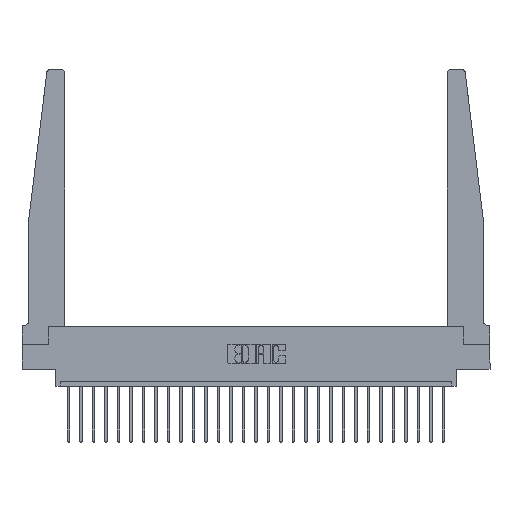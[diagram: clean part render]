
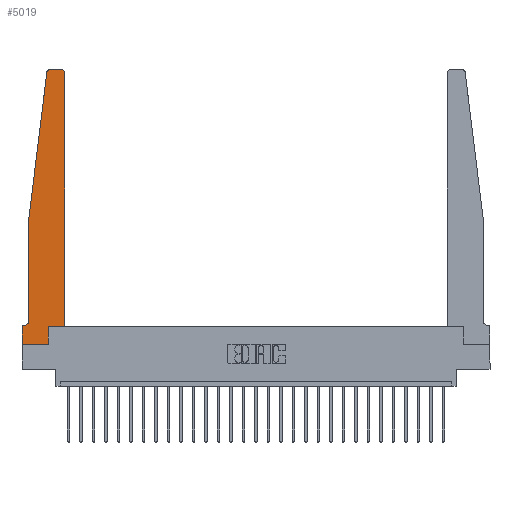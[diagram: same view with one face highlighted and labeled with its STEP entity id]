
A CAD part, top view. The second image highlights one B-rep face of the part: STEP entity #5019.
In plain terms, the highlighted planar face has unit normal (0, 0, 1).
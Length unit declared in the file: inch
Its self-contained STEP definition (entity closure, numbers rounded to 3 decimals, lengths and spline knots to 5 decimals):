
#34 = CARTESIAN_POINT ( 'NONE',  ( 0.065, 1.25, 0.37 ) ) ;
#147 = EDGE_CURVE ( 'NONE', #15718, #2009, #24864, .T. ) ;
#319 = DIRECTION ( 'NONE',  ( 1., 0., 0. ) ) ;
#338 = CARTESIAN_POINT ( 'NONE',  ( 0.425, 0.18, 0.37 ) ) ;
#921 = CARTESIAN_POINT ( 'NONE',  ( 0.2605, 0.18, 0.37 ) ) ;
#945 = EDGE_CURVE ( 'NONE', #9251, #15557, #10658, .T. ) ;
#1356 = VERTEX_POINT ( 'NONE', #6340 ) ;
#1783 = CARTESIAN_POINT ( 'NONE',  ( 0.395, 2.72, 0.37 ) ) ;
#2009 = VERTEX_POINT ( 'NONE', #18451 ) ;
#2066 = CARTESIAN_POINT ( 'NONE',  ( 0., 0., 0.37 ) ) ;
#2299 = DIRECTION ( 'NONE',  ( 0., 1., 0. ) ) ;
#2310 = AXIS2_PLACEMENT_3D ( 'NONE', #1783, #15769, #21494 ) ;
#2678 = EDGE_CURVE ( 'NONE', #15557, #17619, #13947, .T. ) ;
#3442 = EDGE_CURVE ( 'NONE', #2009, #15219, #23476, .T. ) ;
#3740 = LINE ( 'NONE', #34, #7830 ) ;
#4652 = VERTEX_POINT ( 'NONE', #17534 ) ;
#5019 = ADVANCED_FACE ( 'NONE', ( #23372 ), #10019, .T. ) ;
#5149 = VECTOR ( 'NONE', #2299, 39.37008 ) ;
#5150 = CARTESIAN_POINT ( 'NONE',  ( 0.2605, 0.18, 0.37 ) ) ;
#5311 = CARTESIAN_POINT ( 'NONE',  ( 0.015, 0.2375, 0.37 ) ) ;
#5562 = DIRECTION ( 'NONE',  ( 0., -1., 0. ) ) ;
#5778 = CARTESIAN_POINT ( 'NONE',  ( 0.2605, 0., 0.37 ) ) ;
#6340 = CARTESIAN_POINT ( 'NONE',  ( 0.015, 0.1875, 0.37 ) ) ;
#6623 = ORIENTED_EDGE ( 'NONE', *, *, #3442, .T. ) ;
#6877 = VECTOR ( 'NONE', #22052, 39.37008 ) ;
#6918 = CARTESIAN_POINT ( 'NONE',  ( 0.24675, 2.72367, 0.37 ) ) ;
#7830 = VECTOR ( 'NONE', #21625, 39.37008 ) ;
#8407 = ORIENTED_EDGE ( 'NONE', *, *, #9617, .T. ) ;
#8444 = ORIENTED_EDGE ( 'NONE', *, *, #14820, .T. ) ;
#8614 = VECTOR ( 'NONE', #23324, 39.37008 ) ;
#8961 = CIRCLE ( 'NONE', #15081, 0.03 ) ;
#9251 = VERTEX_POINT ( 'NONE', #17848 ) ;
#9331 = VERTEX_POINT ( 'NONE', #10132 ) ;
#9617 = EDGE_CURVE ( 'NONE', #18121, #9331, #22500, .T. ) ;
#9784 = CARTESIAN_POINT ( 'NONE',  ( 0., 0., 0.37 ) ) ;
#9858 = ORIENTED_EDGE ( 'NONE', *, *, #20325, .T. ) ;
#10019 = PLANE ( 'NONE',  #12121 ) ;
#10081 = DIRECTION ( 'NONE',  ( -1., 0., 0. ) ) ;
#10132 = CARTESIAN_POINT ( 'NONE',  ( 0.065, 0.2375, 0.37 ) ) ;
#10326 = CARTESIAN_POINT ( 'NONE',  ( 0.065, 0.1875, 0.37 ) ) ;
#10343 = LINE ( 'NONE', #24431, #23898 ) ;
#10490 = CIRCLE ( 'NONE', #2310, 0.03 ) ;
#10658 = LINE ( 'NONE', #2066, #15305 ) ;
#10981 = ORIENTED_EDGE ( 'NONE', *, *, #12804, .T. ) ;
#11091 = DIRECTION ( 'NONE',  ( 0., 1., 0. ) ) ;
#12029 = CARTESIAN_POINT ( 'NONE',  ( 0., 0.1875, 0.37 ) ) ;
#12121 = AXIS2_PLACEMENT_3D ( 'NONE', #12029, #14042, #319 ) ;
#12804 = EDGE_CURVE ( 'NONE', #15863, #4652, #10343, .T. ) ;
#12866 = EDGE_CURVE ( 'NONE', #18465, #18121, #3740, .T. ) ;
#13024 = EDGE_CURVE ( 'NONE', #1356, #9251, #24803, .T. ) ;
#13165 = CARTESIAN_POINT ( 'NONE',  ( 0.27653, 2.72, 0.37 ) ) ;
#13483 = DIRECTION ( 'NONE',  ( 0., 0., -1. ) ) ;
#13665 = CARTESIAN_POINT ( 'NONE',  ( 0.065, 1.25, 0.37 ) ) ;
#13947 = LINE ( 'NONE', #9784, #8614 ) ;
#14042 = DIRECTION ( 'NONE',  ( 0., 0., 1. ) ) ;
#14306 = ORIENTED_EDGE ( 'NONE', *, *, #24578, .T. ) ;
#14345 = CARTESIAN_POINT ( 'NONE',  ( 0.395, 2.75, 0.37 ) ) ;
#14661 = VECTOR ( 'NONE', #20088, 39.37008 ) ;
#14820 = EDGE_CURVE ( 'NONE', #9331, #1356, #14877, .T. ) ;
#14877 = CIRCLE ( 'NONE', #23794, 0.05 ) ;
#14976 = DIRECTION ( 'NONE',  ( 0., 0., 1. ) ) ;
#15081 = AXIS2_PLACEMENT_3D ( 'NONE', #13165, #14976, #24588 ) ;
#15219 = VERTEX_POINT ( 'NONE', #16617 ) ;
#15278 = EDGE_CURVE ( 'NONE', #4652, #18465, #8961, .T. ) ;
#15305 = VECTOR ( 'NONE', #16053, 39.37008 ) ;
#15557 = VERTEX_POINT ( 'NONE', #18737 ) ;
#15718 = VERTEX_POINT ( 'NONE', #5150 ) ;
#15769 = DIRECTION ( 'NONE',  ( 0., 0., 1. ) ) ;
#15863 = VERTEX_POINT ( 'NONE', #14345 ) ;
#16053 = DIRECTION ( 'NONE',  ( 0., -1., 0. ) ) ;
#16617 = CARTESIAN_POINT ( 'NONE',  ( 0.425, 2.72, 0.37 ) ) ;
#17170 = EDGE_LOOP ( 'NONE', ( #10981, #18918, #18441, #8407, #8444, #24070, #21725, #21412, #9858, #20724, #6623, #14306 ) ) ;
#17534 = CARTESIAN_POINT ( 'NONE',  ( 0.27653, 2.75, 0.37 ) ) ;
#17619 = VERTEX_POINT ( 'NONE', #5778 ) ;
#17848 = CARTESIAN_POINT ( 'NONE',  ( 0., 0.1875, 0.37 ) ) ;
#18121 = VERTEX_POINT ( 'NONE', #21440 ) ;
#18441 = ORIENTED_EDGE ( 'NONE', *, *, #12866, .T. ) ;
#18451 = CARTESIAN_POINT ( 'NONE',  ( 0.425, 0.18, 0.37 ) ) ;
#18465 = VERTEX_POINT ( 'NONE', #6918 ) ;
#18737 = CARTESIAN_POINT ( 'NONE',  ( 0., 0., 0.37 ) ) ;
#18918 = ORIENTED_EDGE ( 'NONE', *, *, #15278, .T. ) ;
#19005 = DIRECTION ( 'NONE',  ( -1., 0., 0. ) ) ;
#19996 = CARTESIAN_POINT ( 'NONE',  ( 0.425, 0.18, 0.37 ) ) ;
#20035 = VECTOR ( 'NONE', #5562, 39.37008 ) ;
#20088 = DIRECTION ( 'NONE',  ( -1., 0., 0. ) ) ;
#20325 = EDGE_CURVE ( 'NONE', #17619, #15718, #22089, .T. ) ;
#20724 = ORIENTED_EDGE ( 'NONE', *, *, #147, .T. ) ;
#21412 = ORIENTED_EDGE ( 'NONE', *, *, #2678, .T. ) ;
#21440 = CARTESIAN_POINT ( 'NONE',  ( 0.065, 1.25, 0.37 ) ) ;
#21494 = DIRECTION ( 'NONE',  ( 1., 0., 0. ) ) ;
#21625 = DIRECTION ( 'NONE',  ( -0.122, -0.992, 0. ) ) ;
#21725 = ORIENTED_EDGE ( 'NONE', *, *, #945, .T. ) ;
#22052 = DIRECTION ( 'NONE',  ( 1., 0., 0. ) ) ;
#22089 = LINE ( 'NONE', #921, #25156 ) ;
#22500 = LINE ( 'NONE', #13665, #20035 ) ;
#23324 = DIRECTION ( 'NONE',  ( 1., 0., 0. ) ) ;
#23372 = FACE_OUTER_BOUND ( 'NONE', #17170, .T. ) ;
#23476 = LINE ( 'NONE', #338, #5149 ) ;
#23794 = AXIS2_PLACEMENT_3D ( 'NONE', #5311, #13483, #10081 ) ;
#23898 = VECTOR ( 'NONE', #19005, 39.37008 ) ;
#24070 = ORIENTED_EDGE ( 'NONE', *, *, #13024, .T. ) ;
#24431 = CARTESIAN_POINT ( 'NONE',  ( 0.25, 2.75, 0.37 ) ) ;
#24578 = EDGE_CURVE ( 'NONE', #15219, #15863, #10490, .T. ) ;
#24588 = DIRECTION ( 'NONE',  ( 1., 0., 0. ) ) ;
#24803 = LINE ( 'NONE', #10326, #14661 ) ;
#24864 = LINE ( 'NONE', #19996, #6877 ) ;
#25156 = VECTOR ( 'NONE', #11091, 39.37008 ) ;
